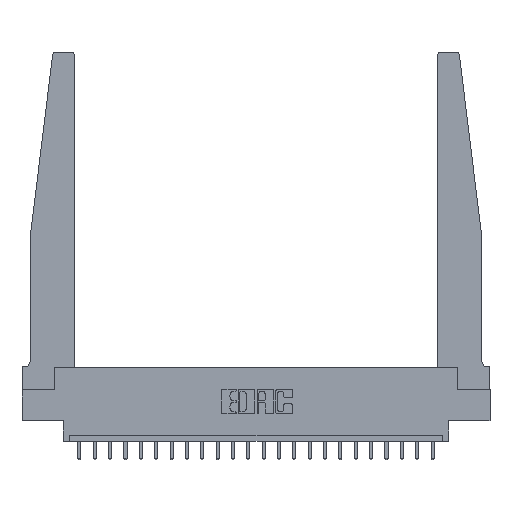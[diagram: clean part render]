
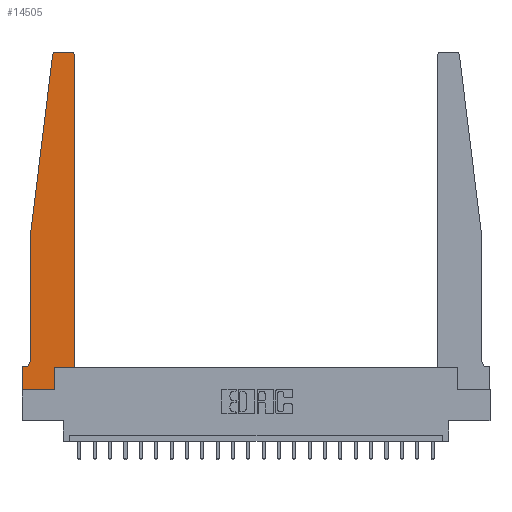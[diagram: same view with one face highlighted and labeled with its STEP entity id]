
A CAD part, top view. The second image highlights one B-rep face of the part: STEP entity #14505.
In plain terms, the highlighted planar face has unit normal (0, 0, 1).
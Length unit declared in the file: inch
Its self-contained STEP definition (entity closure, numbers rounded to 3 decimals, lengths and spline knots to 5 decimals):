
#2 = VECTOR ( 'NONE', #14728, 39.37008 ) ;
#93 = FACE_OUTER_BOUND ( 'NONE', #19054, .T. ) ;
#543 = CARTESIAN_POINT ( 'NONE',  ( 0., 0., 0.37 ) ) ;
#572 = CARTESIAN_POINT ( 'NONE',  ( 0.2605, 0., 0.37 ) ) ;
#792 = CARTESIAN_POINT ( 'NONE',  ( 0.425, 0.18, 0.37 ) ) ;
#1134 = EDGE_CURVE ( 'NONE', #7747, #17416, #19344, .T. ) ;
#1140 = CARTESIAN_POINT ( 'NONE',  ( 0.015, 0.2375, 0.37 ) ) ;
#1152 = CARTESIAN_POINT ( 'NONE',  ( 0., 0., 0.37 ) ) ;
#1189 = DIRECTION ( 'NONE',  ( -1., 0., 0. ) ) ;
#1202 = DIRECTION ( 'NONE',  ( 1., 0., 0. ) ) ;
#1544 = ORIENTED_EDGE ( 'NONE', *, *, #18665, .T. ) ;
#1689 = VECTOR ( 'NONE', #9754, 39.37008 ) ;
#2202 = ORIENTED_EDGE ( 'NONE', *, *, #10784, .T. ) ;
#2291 = VECTOR ( 'NONE', #1189, 39.37008 ) ;
#2420 = AXIS2_PLACEMENT_3D ( 'NONE', #16603, #18260, #19915 ) ;
#2907 = LINE ( 'NONE', #19423, #9293 ) ;
#2982 = AXIS2_PLACEMENT_3D ( 'NONE', #1140, #17940, #20492 ) ;
#3014 = PLANE ( 'NONE',  #2420 ) ;
#3196 = ORIENTED_EDGE ( 'NONE', *, *, #12125, .T. ) ;
#3443 = CARTESIAN_POINT ( 'NONE',  ( 0., 0.1875, 0.37 ) ) ;
#3486 = VERTEX_POINT ( 'NONE', #21038 ) ;
#3671 = DIRECTION ( 'NONE',  ( 1., 0., 0. ) ) ;
#4264 = DIRECTION ( 'NONE',  ( -1., 0., 0. ) ) ;
#4285 = VERTEX_POINT ( 'NONE', #10044 ) ;
#4445 = EDGE_CURVE ( 'NONE', #4285, #14736, #20290, .T. ) ;
#4484 = CARTESIAN_POINT ( 'NONE',  ( 0.425, 2.72, 0.37 ) ) ;
#4521 = EDGE_CURVE ( 'NONE', #3486, #14120, #11959, .T. ) ;
#4996 = DIRECTION ( 'NONE',  ( 0., -1., 0. ) ) ;
#5284 = VERTEX_POINT ( 'NONE', #572 ) ;
#5493 = ORIENTED_EDGE ( 'NONE', *, *, #4521, .T. ) ;
#5504 = CARTESIAN_POINT ( 'NONE',  ( 0.2605, 0.18, 0.37 ) ) ;
#5621 = CARTESIAN_POINT ( 'NONE',  ( 0.425, 0.18, 0.37 ) ) ;
#5823 = DIRECTION ( 'NONE',  ( 1., 0., 0. ) ) ;
#6725 = ORIENTED_EDGE ( 'NONE', *, *, #19170, .T. ) ;
#6985 = LINE ( 'NONE', #9696, #2 ) ;
#7747 = VERTEX_POINT ( 'NONE', #13787 ) ;
#7977 = CARTESIAN_POINT ( 'NONE',  ( 0.27653, 2.72, 0.37 ) ) ;
#8120 = ORIENTED_EDGE ( 'NONE', *, *, #13741, .T. ) ;
#8500 = ORIENTED_EDGE ( 'NONE', *, *, #12212, .T. ) ;
#9267 = CARTESIAN_POINT ( 'NONE',  ( 0.395, 2.75, 0.37 ) ) ;
#9293 = VECTOR ( 'NONE', #4264, 39.37008 ) ;
#9690 = EDGE_CURVE ( 'NONE', #11728, #10366, #9707, .T. ) ;
#9696 = CARTESIAN_POINT ( 'NONE',  ( 0.065, 1.25, 0.37 ) ) ;
#9707 = LINE ( 'NONE', #12044, #20466 ) ;
#9715 = DIRECTION ( 'NONE',  ( 1., 0., 0. ) ) ;
#9754 = DIRECTION ( 'NONE',  ( 0., -1., 0. ) ) ;
#9875 = ORIENTED_EDGE ( 'NONE', *, *, #22167, .T. ) ;
#10017 = AXIS2_PLACEMENT_3D ( 'NONE', #7977, #16410, #9715 ) ;
#10044 = CARTESIAN_POINT ( 'NONE',  ( 0.015, 0.1875, 0.37 ) ) ;
#10366 = VERTEX_POINT ( 'NONE', #20443 ) ;
#10446 = DIRECTION ( 'NONE',  ( 0., 0., 1. ) ) ;
#10661 = LINE ( 'NONE', #5504, #19836 ) ;
#10708 = CARTESIAN_POINT ( 'NONE',  ( 0., 0., 0.37 ) ) ;
#10784 = EDGE_CURVE ( 'NONE', #14198, #5284, #17990, .T. ) ;
#10972 = CARTESIAN_POINT ( 'NONE',  ( 0.065, 1.25, 0.37 ) ) ;
#11076 = LINE ( 'NONE', #1152, #1689 ) ;
#11600 = CARTESIAN_POINT ( 'NONE',  ( 0.065, 0.1875, 0.37 ) ) ;
#11728 = VERTEX_POINT ( 'NONE', #10972 ) ;
#11959 = CIRCLE ( 'NONE', #10017, 0.03 ) ;
#12044 = CARTESIAN_POINT ( 'NONE',  ( 0.065, 1.25, 0.37 ) ) ;
#12125 = EDGE_CURVE ( 'NONE', #17472, #3486, #2907, .T. ) ;
#12212 = EDGE_CURVE ( 'NONE', #10366, #4285, #19533, .T. ) ;
#12499 = CIRCLE ( 'NONE', #17942, 0.03 ) ;
#12987 = CARTESIAN_POINT ( 'NONE',  ( 0.425, 0.18, 0.37 ) ) ;
#13411 = VECTOR ( 'NONE', #3671, 39.37008 ) ;
#13741 = EDGE_CURVE ( 'NONE', #13913, #17472, #12499, .T. ) ;
#13787 = CARTESIAN_POINT ( 'NONE',  ( 0.2605, 0.18, 0.37 ) ) ;
#13913 = VERTEX_POINT ( 'NONE', #4484 ) ;
#14120 = VERTEX_POINT ( 'NONE', #15335 ) ;
#14136 = ORIENTED_EDGE ( 'NONE', *, *, #19564, .T. ) ;
#14198 = VERTEX_POINT ( 'NONE', #543 ) ;
#14374 = DIRECTION ( 'NONE',  ( 0., 1., 0. ) ) ;
#14505 = ADVANCED_FACE ( 'NONE', ( #93 ), #3014, .T. ) ;
#14728 = DIRECTION ( 'NONE',  ( -0.122, -0.992, 0. ) ) ;
#14736 = VERTEX_POINT ( 'NONE', #3443 ) ;
#15335 = CARTESIAN_POINT ( 'NONE',  ( 0.24675, 2.72367, 0.37 ) ) ;
#15642 = CARTESIAN_POINT ( 'NONE',  ( 0.395, 2.72, 0.37 ) ) ;
#16272 = ORIENTED_EDGE ( 'NONE', *, *, #1134, .T. ) ;
#16410 = DIRECTION ( 'NONE',  ( 0., 0., 1. ) ) ;
#16603 = CARTESIAN_POINT ( 'NONE',  ( 0., 0.1875, 0.37 ) ) ;
#16616 = VECTOR ( 'NONE', #14374, 39.37008 ) ;
#17152 = LINE ( 'NONE', #792, #16616 ) ;
#17195 = VECTOR ( 'NONE', #1202, 39.37008 ) ;
#17416 = VERTEX_POINT ( 'NONE', #5621 ) ;
#17472 = VERTEX_POINT ( 'NONE', #9267 ) ;
#17940 = DIRECTION ( 'NONE',  ( 0., 0., -1. ) ) ;
#17942 = AXIS2_PLACEMENT_3D ( 'NONE', #15642, #10446, #5823 ) ;
#17990 = LINE ( 'NONE', #10708, #13411 ) ;
#18209 = ORIENTED_EDGE ( 'NONE', *, *, #9690, .T. ) ;
#18260 = DIRECTION ( 'NONE',  ( 0., 0., 1. ) ) ;
#18558 = ORIENTED_EDGE ( 'NONE', *, *, #4445, .T. ) ;
#18665 = EDGE_CURVE ( 'NONE', #14120, #11728, #6985, .T. ) ;
#19027 = DIRECTION ( 'NONE',  ( 0., 1., 0. ) ) ;
#19054 = EDGE_LOOP ( 'NONE', ( #3196, #5493, #1544, #18209, #8500, #18558, #9875, #2202, #14136, #16272, #6725, #8120 ) ) ;
#19170 = EDGE_CURVE ( 'NONE', #17416, #13913, #17152, .T. ) ;
#19344 = LINE ( 'NONE', #12987, #17195 ) ;
#19423 = CARTESIAN_POINT ( 'NONE',  ( 0.25, 2.75, 0.37 ) ) ;
#19533 = CIRCLE ( 'NONE', #2982, 0.05 ) ;
#19564 = EDGE_CURVE ( 'NONE', #5284, #7747, #10661, .T. ) ;
#19836 = VECTOR ( 'NONE', #19027, 39.37008 ) ;
#19915 = DIRECTION ( 'NONE',  ( 1., 0., 0. ) ) ;
#20290 = LINE ( 'NONE', #11600, #2291 ) ;
#20443 = CARTESIAN_POINT ( 'NONE',  ( 0.065, 0.2375, 0.37 ) ) ;
#20466 = VECTOR ( 'NONE', #4996, 39.37008 ) ;
#20492 = DIRECTION ( 'NONE',  ( -1., 0., 0. ) ) ;
#21038 = CARTESIAN_POINT ( 'NONE',  ( 0.27653, 2.75, 0.37 ) ) ;
#22167 = EDGE_CURVE ( 'NONE', #14736, #14198, #11076, .T. ) ;
